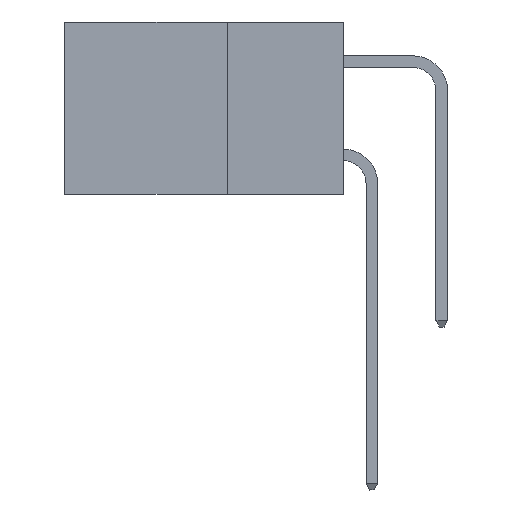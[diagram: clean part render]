
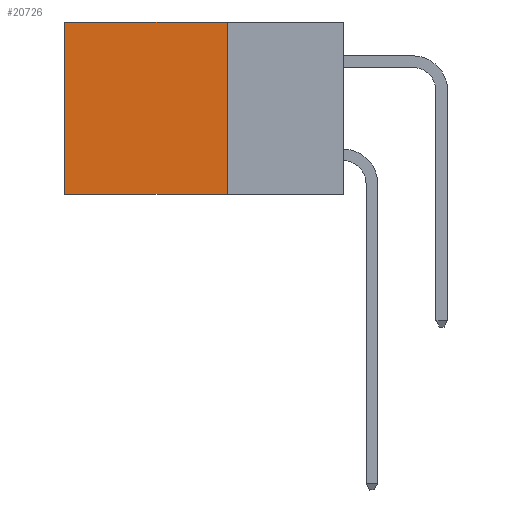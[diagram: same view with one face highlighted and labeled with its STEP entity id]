
A CAD part, left-side view. The second image highlights one B-rep face of the part: STEP entity #20726.
In plain terms, the highlighted planar face has unit normal (-1, 0, 0).
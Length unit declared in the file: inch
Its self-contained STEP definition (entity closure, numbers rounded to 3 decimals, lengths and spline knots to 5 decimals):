
#1213 = DIRECTION ( 'NONE',  ( 0., 1., 0. ) ) ;
#1637 = DIRECTION ( 'NONE',  ( 0., 0., -1. ) ) ;
#1797 = VERTEX_POINT ( 'NONE', #23706 ) ;
#2372 = CARTESIAN_POINT ( 'NONE',  ( 0.2615, 0.25, 0. ) ) ;
#3344 = EDGE_CURVE ( 'NONE', #5231, #21209, #6910, .T. ) ;
#3510 = EDGE_CURVE ( 'NONE', #21209, #7437, #13217, .T. ) ;
#5231 = VERTEX_POINT ( 'NONE', #2372 ) ;
#5887 = EDGE_CURVE ( 'NONE', #5231, #1797, #6402, .T. ) ;
#6204 = VECTOR ( 'NONE', #6949, 39.37008 ) ;
#6402 = LINE ( 'NONE', #7207, #17568 ) ;
#6910 = LINE ( 'NONE', #7197, #6204 ) ;
#6932 = ORIENTED_EDGE ( 'NONE', *, *, #27291, .F. ) ;
#6949 = DIRECTION ( 'NONE',  ( 0., 1., 0. ) ) ;
#7197 = CARTESIAN_POINT ( 'NONE',  ( 0.2615, 0.25, 0. ) ) ;
#7207 = CARTESIAN_POINT ( 'NONE',  ( 0.2615, 0.25, -0.37 ) ) ;
#7244 = VECTOR ( 'NONE', #1637, 39.37008 ) ;
#7437 = VERTEX_POINT ( 'NONE', #14464 ) ;
#8971 = LINE ( 'NONE', #25725, #14252 ) ;
#11547 = ORIENTED_EDGE ( 'NONE', *, *, #3344, .T. ) ;
#11727 = DIRECTION ( 'NONE',  ( 0., 0., -1. ) ) ;
#13149 = CARTESIAN_POINT ( 'NONE',  ( 0.2615, 0.25, -0.37 ) ) ;
#13217 = LINE ( 'NONE', #23929, #7244 ) ;
#14252 = VECTOR ( 'NONE', #1213, 39.37008 ) ;
#14464 = CARTESIAN_POINT ( 'NONE',  ( 0.2615, 0.6, -0.37 ) ) ;
#14481 = AXIS2_PLACEMENT_3D ( 'NONE', #13149, #28542, #15375 ) ;
#15375 = DIRECTION ( 'NONE',  ( 0., 0., -1. ) ) ;
#15682 = EDGE_LOOP ( 'NONE', ( #16285, #6932, #27592, #11547 ) ) ;
#16285 = ORIENTED_EDGE ( 'NONE', *, *, #3510, .T. ) ;
#17568 = VECTOR ( 'NONE', #11727, 39.37008 ) ;
#19024 = CARTESIAN_POINT ( 'NONE',  ( 0.2615, 0.6, 0. ) ) ;
#20726 = ADVANCED_FACE ( 'NONE', ( #28042 ), #24161, .F. ) ;
#21209 = VERTEX_POINT ( 'NONE', #19024 ) ;
#23706 = CARTESIAN_POINT ( 'NONE',  ( 0.2615, 0.25, -0.37 ) ) ;
#23929 = CARTESIAN_POINT ( 'NONE',  ( 0.2615, 0.6, -0.37 ) ) ;
#24161 = PLANE ( 'NONE',  #14481 ) ;
#25725 = CARTESIAN_POINT ( 'NONE',  ( 0.2615, 0.25, -0.37 ) ) ;
#27291 = EDGE_CURVE ( 'NONE', #1797, #7437, #8971, .T. ) ;
#27592 = ORIENTED_EDGE ( 'NONE', *, *, #5887, .F. ) ;
#28042 = FACE_OUTER_BOUND ( 'NONE', #15682, .T. ) ;
#28542 = DIRECTION ( 'NONE',  ( 1., 0., 0. ) ) ;
